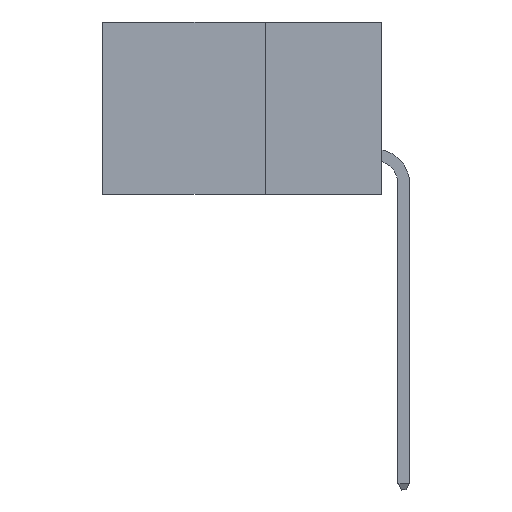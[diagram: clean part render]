
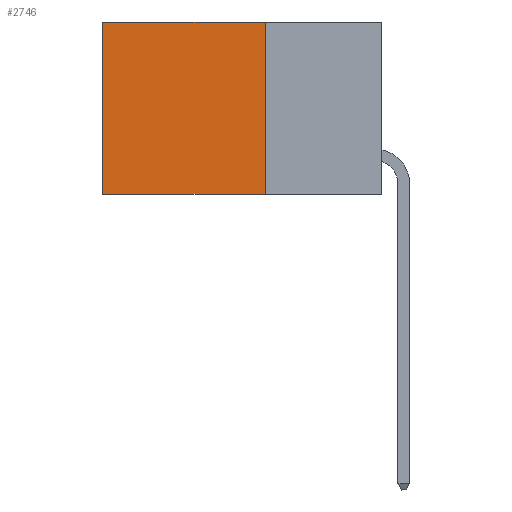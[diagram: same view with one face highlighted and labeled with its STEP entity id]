
A CAD part, left-side view. The second image highlights one B-rep face of the part: STEP entity #2746.
In plain terms, the highlighted planar face has unit normal (-1, 0, 0).
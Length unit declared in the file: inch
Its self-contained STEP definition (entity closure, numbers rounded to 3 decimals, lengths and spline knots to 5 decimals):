
#647 = PLANE ( 'NONE',  #36135 ) ;
#837 = VECTOR ( 'NONE', #17035, 39.37008 ) ;
#1325 = EDGE_CURVE ( 'NONE', #9036, #33641, #23655, .T. ) ;
#2746 = ADVANCED_FACE ( 'NONE', ( #36681 ), #647, .F. ) ;
#2885 = EDGE_LOOP ( 'NONE', ( #21062, #9960, #23461, #16405 ) ) ;
#2897 = VECTOR ( 'NONE', #5757, 39.37008 ) ;
#4318 = VERTEX_POINT ( 'NONE', #41717 ) ;
#5757 = DIRECTION ( 'NONE',  ( 0., 0., -1. ) ) ;
#6223 = EDGE_CURVE ( 'NONE', #33525, #9036, #6957, .T. ) ;
#6957 = LINE ( 'NONE', #12628, #12054 ) ;
#9036 = VERTEX_POINT ( 'NONE', #16474 ) ;
#9960 = ORIENTED_EDGE ( 'NONE', *, *, #1325, .F. ) ;
#12054 = VECTOR ( 'NONE', #45081, 39.37008 ) ;
#12560 = EDGE_CURVE ( 'NONE', #4318, #33641, #15437, .T. ) ;
#12628 = CARTESIAN_POINT ( 'NONE',  ( 0.2875, 0.25, 0. ) ) ;
#13341 = CARTESIAN_POINT ( 'NONE',  ( 0.2875, 0.25, 0. ) ) ;
#15437 = LINE ( 'NONE', #42160, #2897 ) ;
#16155 = CARTESIAN_POINT ( 'NONE',  ( 0.2875, 0.25, -0.37 ) ) ;
#16405 = ORIENTED_EDGE ( 'NONE', *, *, #34894, .T. ) ;
#16474 = CARTESIAN_POINT ( 'NONE',  ( 0.2875, 0.25, -0.37 ) ) ;
#17035 = DIRECTION ( 'NONE',  ( 0., 1., 0. ) ) ;
#17130 = CARTESIAN_POINT ( 'NONE',  ( 0.2875, 0.6, -0.37 ) ) ;
#18625 = DIRECTION ( 'NONE',  ( 1., 0., 0. ) ) ;
#21062 = ORIENTED_EDGE ( 'NONE', *, *, #12560, .T. ) ;
#22517 = VECTOR ( 'NONE', #34730, 39.37008 ) ;
#23461 = ORIENTED_EDGE ( 'NONE', *, *, #6223, .F. ) ;
#23655 = LINE ( 'NONE', #16155, #22517 ) ;
#33525 = VERTEX_POINT ( 'NONE', #34769 ) ;
#33641 = VERTEX_POINT ( 'NONE', #17130 ) ;
#34730 = DIRECTION ( 'NONE',  ( 0., 1., 0. ) ) ;
#34769 = CARTESIAN_POINT ( 'NONE',  ( 0.2875, 0.25, 0. ) ) ;
#34894 = EDGE_CURVE ( 'NONE', #33525, #4318, #40671, .T. ) ;
#36135 = AXIS2_PLACEMENT_3D ( 'NONE', #40086, #18625, #43748 ) ;
#36681 = FACE_OUTER_BOUND ( 'NONE', #2885, .T. ) ;
#40086 = CARTESIAN_POINT ( 'NONE',  ( 0.2875, 0.25, 0. ) ) ;
#40671 = LINE ( 'NONE', #13341, #837 ) ;
#41717 = CARTESIAN_POINT ( 'NONE',  ( 0.2875, 0.6, 0. ) ) ;
#42160 = CARTESIAN_POINT ( 'NONE',  ( 0.2875, 0.6, 0. ) ) ;
#43748 = DIRECTION ( 'NONE',  ( 0., 0., -1. ) ) ;
#45081 = DIRECTION ( 'NONE',  ( 0., 0., -1. ) ) ;
